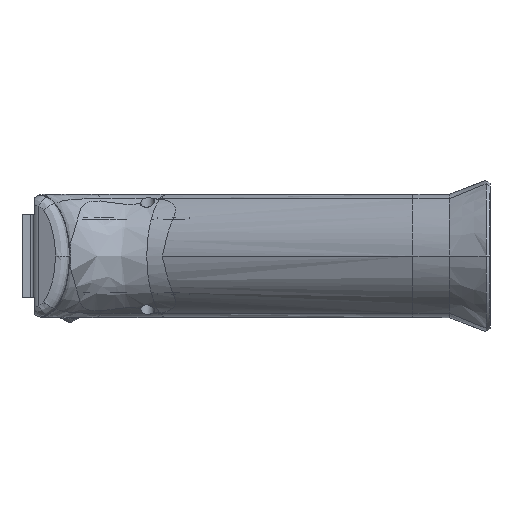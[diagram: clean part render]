
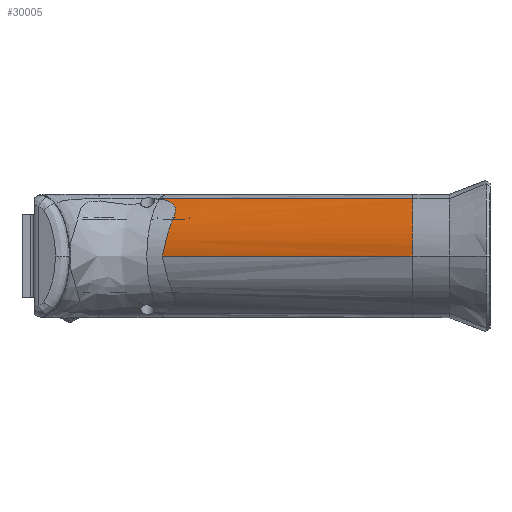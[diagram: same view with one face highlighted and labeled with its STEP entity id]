
A CAD part, left-side view. The second image highlights one B-rep face of the part: STEP entity #30005.
In plain terms, the highlighted free-form (B-spline) face has degree [3, 1] with [18, 2] control points.
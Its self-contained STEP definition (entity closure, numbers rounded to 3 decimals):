
#628=B_SPLINE_SURFACE_WITH_KNOTS('',3,1,((#58120,#58121),(#58122,#58123),
(#58124,#58125),(#58126,#58127),(#58128,#58129),(#58130,#58131),(#58132,
#58133),(#58134,#58135),(#58136,#58137),(#58138,#58139),(#58140,#58141),
(#58142,#58143),(#58144,#58145),(#58146,#58147),(#58148,#58149),(#58150,
#58151),(#58152,#58153),(#58154,#58155)),.UNSPECIFIED.,.F.,.F.,.F.,(4,2,
3,2,2,3,2,4),(2,2),(-6.248,-1.98,-1.702,
-1.223,-0.763,0.,0.061,
0.631),(0.,10.975),.UNSPECIFIED.);
#737=B_SPLINE_CURVE_WITH_KNOTS('',3,(#45908,#45909,#45910,#45911,#45912,
#45913,#45914,#45915,#45916,#45917),.UNSPECIFIED.,.F.,.F.,(4,3,3,4),(-1.733,
-1.263,-0.786,0.),.UNSPECIFIED.);
#987=B_SPLINE_CURVE_WITH_KNOTS('',3,(#58165,#58166,#58167,#58168,#58169,
#58170,#58171,#58172,#58173,#58174,#58175,#58176,#58177,#58178,#58179,#58180,
#58181,#58182,#58183,#58184,#58185,#58186,#58187,#58188,#58189,#58190,#58191,
#58192,#58193,#58194,#58195,#58196,#58197,#58198),.UNSPECIFIED.,.F.,.F.,
(4,2,2,2,2,2,2,2,2,2,2,2,2,2,2,2,4),(-1.724,-1.502,
-1.331,-1.174,-1.094,-1.037,
-0.974,-0.84,-0.535,-0.27,
-0.126,-0.061,-0.03,-0.015,
-0.007,-0.004,0.),
 .UNSPECIFIED.);
#3481=LINE('',#58157,#6668);
#3482=LINE('',#58159,#6669);
#3483=LINE('',#58199,#6670);
#6668=VECTOR('',#37269,10.);
#6669=VECTOR('',#37270,10.);
#6670=VECTOR('',#37275,10.);
#9765=FACE_OUTER_BOUND('',#11530,.T.);
#11530=EDGE_LOOP('',(#25235,#25236,#25237,#25238,#25239,#25240,#25241));
#12377=ELLIPSE('',#31909,163.607,48.254);
#12721=CIRCLE('',#31910,2.686);
#14378=VERTEX_POINT('',#45873);
#14379=VERTEX_POINT('',#45907);
#15029=VERTEX_POINT('',#58156);
#15030=VERTEX_POINT('',#58158);
#15031=VERTEX_POINT('',#58160);
#15032=VERTEX_POINT('',#58162);
#15033=VERTEX_POINT('',#58164);
#17766=EDGE_CURVE('',#14378,#14379,#737,.T.);
#18726=EDGE_CURVE('',#15029,#14379,#3481,.T.);
#18727=EDGE_CURVE('',#15030,#15029,#3482,.T.);
#18728=EDGE_CURVE('',#15031,#15030,#12377,.T.);
#18729=EDGE_CURVE('',#15031,#15032,#12721,.T.);
#18730=EDGE_CURVE('',#15032,#15033,#987,.T.);
#18731=EDGE_CURVE('',#15033,#14378,#3483,.T.);
#25235=ORIENTED_EDGE('',*,*,#17766,.T.);
#25236=ORIENTED_EDGE('',*,*,#18726,.F.);
#25237=ORIENTED_EDGE('',*,*,#18727,.F.);
#25238=ORIENTED_EDGE('',*,*,#18728,.F.);
#25239=ORIENTED_EDGE('',*,*,#18729,.T.);
#25240=ORIENTED_EDGE('',*,*,#18730,.T.);
#25241=ORIENTED_EDGE('',*,*,#18731,.T.);
#30005=ADVANCED_FACE('',(#9765),#628,.F.);
#31909=AXIS2_PLACEMENT_3D('',#58161,#37271,#37272);
#31910=AXIS2_PLACEMENT_3D('',#58163,#37273,#37274);
#37269=DIRECTION('',(-0.367,-0.93,0.));
#37270=DIRECTION('',(-0.367,-0.93,0.));
#37271=DIRECTION('center_axis',(0.367,0.93,0.));
#37272=DIRECTION('ref_axis',(0.877,-0.345,-0.335));
#37273=DIRECTION('center_axis',(-0.475,0.299,0.828));
#37274=DIRECTION('ref_axis',(-0.393,-0.914,0.105));
#37275=DIRECTION('',(-0.367,-0.93,0.));
#45873=CARTESIAN_POINT('',(-11.371,-89.732,0.));
#45907=CARTESIAN_POINT('',(-2.674,-89.732,13.366));
#45908=CARTESIAN_POINT('Ctrl Pts',(-11.371,-89.732,
0.));
#45909=CARTESIAN_POINT('Ctrl Pts',(-11.315,-89.732,
1.426));
#45910=CARTESIAN_POINT('Ctrl Pts',(-11.07,-89.732,
2.844));
#45911=CARTESIAN_POINT('Ctrl Pts',(-10.615,-89.732,
4.197));
#45912=CARTESIAN_POINT('Ctrl Pts',(-10.152,-89.732,
5.573));
#45913=CARTESIAN_POINT('Ctrl Pts',(-9.467,-89.732,
6.903));
#45914=CARTESIAN_POINT('Ctrl Pts',(-8.523,-89.732,
8.186));
#45915=CARTESIAN_POINT('Ctrl Pts',(-6.971,-89.732,10.295));
#45916=CARTESIAN_POINT('Ctrl Pts',(-4.905,-89.732,
11.995));
#45917=CARTESIAN_POINT('Ctrl Pts',(-2.674,-89.732,13.366));
#58120=CARTESIAN_POINT('Ctrl Pts',(11.945,-27.357,-45.174));
#58121=CARTESIAN_POINT('Ctrl Pts',(-28.278,-129.47,
-45.174));
#58122=CARTESIAN_POINT('Ctrl Pts',(12.253,-27.479,-32.36));
#58123=CARTESIAN_POINT('Ctrl Pts',(-27.97,-129.592,
-32.36));
#58124=CARTESIAN_POINT('Ctrl Pts',(12.561,-27.6,-19.535));
#58125=CARTESIAN_POINT('Ctrl Pts',(-27.662,-129.713,
-19.535));
#58126=CARTESIAN_POINT('Ctrl Pts',(12.889,-27.729,-5.885));
#58127=CARTESIAN_POINT('Ctrl Pts',(-27.335,-129.842,
-5.885));
#58128=CARTESIAN_POINT('Ctrl Pts',(13.003,-27.774,-0.836));
#58129=CARTESIAN_POINT('Ctrl Pts',(-27.221,-129.887,-0.836));
#58130=CARTESIAN_POINT('Ctrl Pts',(13.031,-27.785,0.));
#58131=CARTESIAN_POINT('Ctrl Pts',(-27.193,-129.898,
0.));
#58132=CARTESIAN_POINT('Ctrl Pts',(13.079,-27.804,1.437));
#58133=CARTESIAN_POINT('Ctrl Pts',(-27.144,-129.917,
1.437));
#58134=CARTESIAN_POINT('Ctrl Pts',(13.295,-27.889,2.877));
#58135=CARTESIAN_POINT('Ctrl Pts',(-26.929,-130.002,
2.877));
#58136=CARTESIAN_POINT('Ctrl Pts',(14.093,-28.203,5.579));
#58137=CARTESIAN_POINT('Ctrl Pts',(-26.13,-130.317,
5.579));
#58138=CARTESIAN_POINT('Ctrl Pts',(14.667,-28.429,6.876));
#58139=CARTESIAN_POINT('Ctrl Pts',(-25.557,-130.542,
6.876));
#58140=CARTESIAN_POINT('Ctrl Pts',(16.802,-29.27,10.249));
#58141=CARTESIAN_POINT('Ctrl Pts',(-23.422,-131.383,
10.249));
#58142=CARTESIAN_POINT('Ctrl Pts',(18.586,-29.973,11.965));
#58143=CARTESIAN_POINT('Ctrl Pts',(-21.638,-132.086,
11.965));
#58144=CARTESIAN_POINT('Ctrl Pts',(20.559,-30.75,13.366));
#58145=CARTESIAN_POINT('Ctrl Pts',(-19.664,-132.864,
13.366));
#58146=CARTESIAN_POINT('Ctrl Pts',(20.717,-30.812,13.478));
#58147=CARTESIAN_POINT('Ctrl Pts',(-19.507,-132.926,
13.478));
#58148=CARTESIAN_POINT('Ctrl Pts',(20.893,-30.882,13.601));
#58149=CARTESIAN_POINT('Ctrl Pts',(-19.331,-132.995,
13.601));
#58150=CARTESIAN_POINT('Ctrl Pts',(22.534,-31.528,14.749));
#58151=CARTESIAN_POINT('Ctrl Pts',(-17.69,-133.641,14.749));
#58152=CARTESIAN_POINT('Ctrl Pts',(24.028,-32.117,15.797));
#58153=CARTESIAN_POINT('Ctrl Pts',(-16.196,-134.23,
15.797));
#58154=CARTESIAN_POINT('Ctrl Pts',(25.508,-32.7,16.838));
#58155=CARTESIAN_POINT('Ctrl Pts',(-14.715,-134.813,
16.838));
#58156=CARTESIAN_POINT('',(20.434,-31.067,13.366));
#58157=CARTESIAN_POINT('',(20.555,-30.76,13.366));
#58158=CARTESIAN_POINT('',(20.555,-30.76,13.366));
#58159=CARTESIAN_POINT('',(20.555,-30.76,13.366));
#58160=CARTESIAN_POINT('',(20.41,-30.703,13.263));
#58161=CARTESIAN_POINT('Origin',(157.307,-84.628,-50.021));
#58162=CARTESIAN_POINT('',(20.555,-30.76,13.366));
#58163=CARTESIAN_POINT('Origin',(21.61,-28.306,13.085));
#58164=CARTESIAN_POINT('',(11.685,-31.202,0.));
#58165=CARTESIAN_POINT('Ctrl Pts',(20.555,-30.76,13.366));
#58166=CARTESIAN_POINT('Ctrl Pts',(20.079,-31.393,13.227));
#58167=CARTESIAN_POINT('Ctrl Pts',(19.552,-32.029,13.053));
#58168=CARTESIAN_POINT('Ctrl Pts',(18.578,-33.,12.659));
#58169=CARTESIAN_POINT('Ctrl Pts',(18.118,-33.393,12.449));
#58170=CARTESIAN_POINT('Ctrl Pts',(17.199,-33.973,11.942));
#58171=CARTESIAN_POINT('Ctrl Pts',(16.753,-34.168,11.659));
#58172=CARTESIAN_POINT('Ctrl Pts',(16.071,-34.303,11.134));
#58173=CARTESIAN_POINT('Ctrl Pts',(15.848,-34.32,10.945));
#58174=CARTESIAN_POINT('Ctrl Pts',(15.477,-34.305,10.603));
#58175=CARTESIAN_POINT('Ctrl Pts',(15.33,-34.287,10.457));
#58176=CARTESIAN_POINT('Ctrl Pts',(15.028,-34.228,10.141));
#58177=CARTESIAN_POINT('Ctrl Pts',(14.877,-34.184,9.971));
#58178=CARTESIAN_POINT('Ctrl Pts',(14.427,-34.025,9.432));
#58179=CARTESIAN_POINT('Ctrl Pts',(14.149,-33.879,9.048));
#58180=CARTESIAN_POINT('Ctrl Pts',(13.323,-33.376,7.76));
#58181=CARTESIAN_POINT('Ctrl Pts',(12.82,-32.938,6.722));
#58182=CARTESIAN_POINT('Ctrl Pts',(12.061,-32.249,4.441));
#58183=CARTESIAN_POINT('Ctrl Pts',(11.858,-32.044,3.466));
#58184=CARTESIAN_POINT('Ctrl Pts',(11.691,-31.756,2.146));
#58185=CARTESIAN_POINT('Ctrl Pts',(11.656,-31.652,1.681));
#58186=CARTESIAN_POINT('Ctrl Pts',(11.643,-31.484,1.005));
#58187=CARTESIAN_POINT('Ctrl Pts',(11.645,-31.429,0.794));
#58188=CARTESIAN_POINT('Ctrl Pts',(11.655,-31.344,0.484));
#58189=CARTESIAN_POINT('Ctrl Pts',(11.659,-31.316,0.384));
#58190=CARTESIAN_POINT('Ctrl Pts',(11.668,-31.273,0.237));
#58191=CARTESIAN_POINT('Ctrl Pts',(11.671,-31.259,0.189));
#58192=CARTESIAN_POINT('Ctrl Pts',(11.676,-31.238,0.118));
#58193=CARTESIAN_POINT('Ctrl Pts',(11.677,-31.231,0.094));
#58194=CARTESIAN_POINT('Ctrl Pts',(11.68,-31.22,0.058));
#58195=CARTESIAN_POINT('Ctrl Pts',(11.681,-31.216,0.047));
#58196=CARTESIAN_POINT('Ctrl Pts',(11.683,-31.209,0.023));
#58197=CARTESIAN_POINT('Ctrl Pts',(11.684,-31.206,0.012));
#58198=CARTESIAN_POINT('Ctrl Pts',(11.685,-31.202,0.));
#58199=CARTESIAN_POINT('',(13.027,-27.794,0.));
